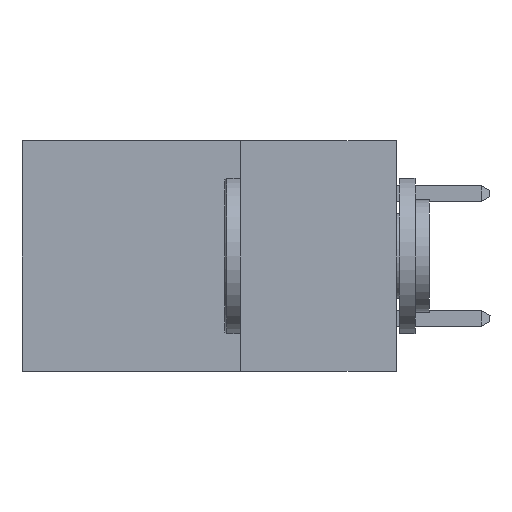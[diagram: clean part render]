
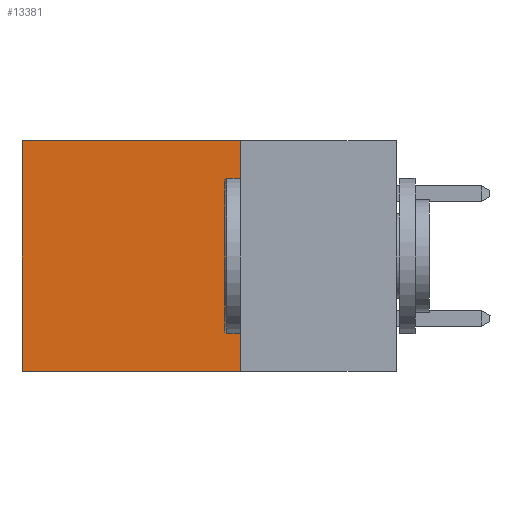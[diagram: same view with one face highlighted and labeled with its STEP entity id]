
A CAD part, left-side view. The second image highlights one B-rep face of the part: STEP entity #13381.
In plain terms, the highlighted planar face has unit normal (-1, 0, 0).
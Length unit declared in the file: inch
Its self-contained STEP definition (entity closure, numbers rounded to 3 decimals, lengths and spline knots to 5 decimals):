
#927 = AXIS2_PLACEMENT_3D ( 'NONE', #18652, #5656, #17129 ) ;
#1221 = DIRECTION ( 'NONE',  ( 0., 1., 0. ) ) ;
#1962 = LINE ( 'NONE', #20709, #5284 ) ;
#2920 = VERTEX_POINT ( 'NONE', #20429 ) ;
#3592 = LINE ( 'NONE', #9562, #6925 ) ;
#5284 = VECTOR ( 'NONE', #20464, 39.37008 ) ;
#5656 = DIRECTION ( 'NONE',  ( 1., 0., 0. ) ) ;
#5872 = CARTESIAN_POINT ( 'NONE',  ( 0.2615, 0.6, -0.37 ) ) ;
#6925 = VECTOR ( 'NONE', #1221, 39.37008 ) ;
#7266 = PLANE ( 'NONE',  #927 ) ;
#7275 = EDGE_CURVE ( 'NONE', #7576, #11235, #1962, .T. ) ;
#7576 = VERTEX_POINT ( 'NONE', #16696 ) ;
#7702 = DIRECTION ( 'NONE',  ( 0., 0., -1. ) ) ;
#7722 = CARTESIAN_POINT ( 'NONE',  ( 0.2615, 0.6, -0.37 ) ) ;
#8256 = DIRECTION ( 'NONE',  ( 0., 0., -1. ) ) ;
#8348 = EDGE_CURVE ( 'NONE', #11235, #18772, #18999, .T. ) ;
#8561 = VECTOR ( 'NONE', #8256, 39.37008 ) ;
#8756 = ORIENTED_EDGE ( 'NONE', *, *, #7275, .T. ) ;
#8830 = ORIENTED_EDGE ( 'NONE', *, *, #20962, .F. ) ;
#9562 = CARTESIAN_POINT ( 'NONE',  ( 0.2615, 0.25, -0.37 ) ) ;
#10445 = VECTOR ( 'NONE', #7702, 39.37008 ) ;
#11235 = VERTEX_POINT ( 'NONE', #13548 ) ;
#11482 = FACE_OUTER_BOUND ( 'NONE', #13925, .T. ) ;
#11547 = EDGE_CURVE ( 'NONE', #2920, #18772, #3592, .T. ) ;
#11598 = CARTESIAN_POINT ( 'NONE',  ( 0.2615, 0.25, -0.37 ) ) ;
#13381 = ADVANCED_FACE ( 'NONE', ( #11482 ), #7266, .F. ) ;
#13548 = CARTESIAN_POINT ( 'NONE',  ( 0.2615, 0.6, 0. ) ) ;
#13925 = EDGE_LOOP ( 'NONE', ( #14980, #16260, #8830, #8756 ) ) ;
#14980 = ORIENTED_EDGE ( 'NONE', *, *, #8348, .T. ) ;
#16260 = ORIENTED_EDGE ( 'NONE', *, *, #11547, .F. ) ;
#16696 = CARTESIAN_POINT ( 'NONE',  ( 0.2615, 0.25, 0. ) ) ;
#17129 = DIRECTION ( 'NONE',  ( 0., 0., -1. ) ) ;
#17731 = LINE ( 'NONE', #11598, #8561 ) ;
#18652 = CARTESIAN_POINT ( 'NONE',  ( 0.2615, 0.25, -0.37 ) ) ;
#18772 = VERTEX_POINT ( 'NONE', #5872 ) ;
#18999 = LINE ( 'NONE', #7722, #10445 ) ;
#20429 = CARTESIAN_POINT ( 'NONE',  ( 0.2615, 0.25, -0.37 ) ) ;
#20464 = DIRECTION ( 'NONE',  ( 0., 1., 0. ) ) ;
#20709 = CARTESIAN_POINT ( 'NONE',  ( 0.2615, 0.25, 0. ) ) ;
#20962 = EDGE_CURVE ( 'NONE', #7576, #2920, #17731, .T. ) ;
